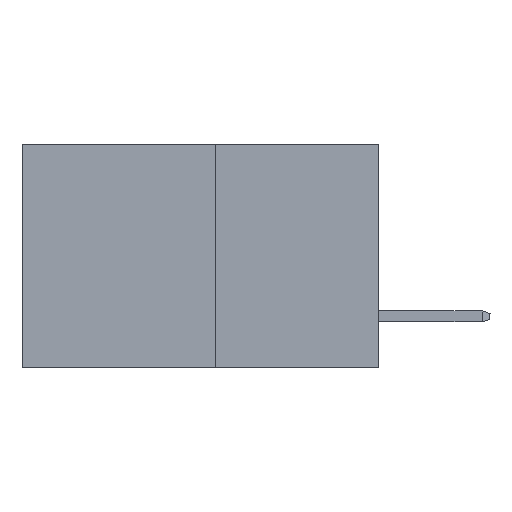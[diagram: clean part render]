
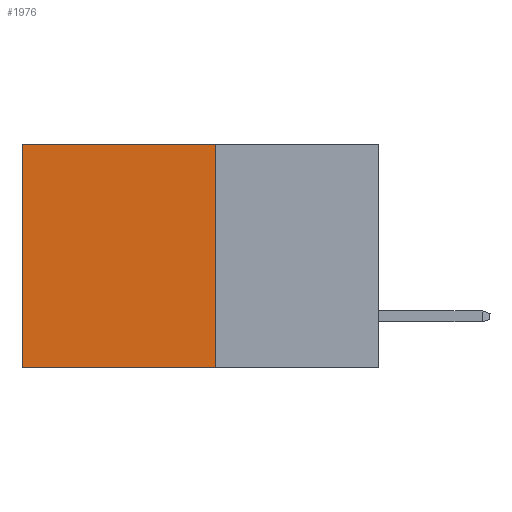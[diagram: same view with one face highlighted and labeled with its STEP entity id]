
A CAD part, left-side view. The second image highlights one B-rep face of the part: STEP entity #1976.
In plain terms, the highlighted planar face has unit normal (-1, 0, 0).
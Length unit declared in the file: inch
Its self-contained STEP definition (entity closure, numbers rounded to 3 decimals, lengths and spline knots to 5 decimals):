
#102 = AXIS2_PLACEMENT_3D ( 'NONE', #6379, #11119, #2765 ) ;
#424 = DIRECTION ( 'NONE',  ( 0., 0., -1. ) ) ;
#978 = VECTOR ( 'NONE', #2847, 39.37008 ) ;
#984 = EDGE_CURVE ( 'NONE', #10551, #9111, #11669, .T. ) ;
#1069 = VECTOR ( 'NONE', #6857, 39.37008 ) ;
#1728 = EDGE_LOOP ( 'NONE', ( #4679, #6504, #8886, #12723 ) ) ;
#1844 = VECTOR ( 'NONE', #10695, 39.37008 ) ;
#1976 = ADVANCED_FACE ( 'NONE', ( #5965 ), #11493, .F. ) ;
#2765 = DIRECTION ( 'NONE',  ( 0., 0., -1. ) ) ;
#2815 = LINE ( 'NONE', #11566, #1844 ) ;
#2847 = DIRECTION ( 'NONE',  ( 0., 1., 0. ) ) ;
#3214 = EDGE_CURVE ( 'NONE', #10551, #5088, #2815, .T. ) ;
#4679 = ORIENTED_EDGE ( 'NONE', *, *, #10017, .T. ) ;
#4968 = CARTESIAN_POINT ( 'NONE',  ( 0.277, 0.59, -0.37 ) ) ;
#5088 = VERTEX_POINT ( 'NONE', #12902 ) ;
#5836 = CARTESIAN_POINT ( 'NONE',  ( 0.277, 0.27, -0.37 ) ) ;
#5965 = FACE_OUTER_BOUND ( 'NONE', #1728, .T. ) ;
#6203 = CARTESIAN_POINT ( 'NONE',  ( 0.277, 0.59, 0. ) ) ;
#6379 = CARTESIAN_POINT ( 'NONE',  ( 0.277, 0.27, -0.37 ) ) ;
#6504 = ORIENTED_EDGE ( 'NONE', *, *, #12082, .F. ) ;
#6857 = DIRECTION ( 'NONE',  ( 0., 1., 0. ) ) ;
#8818 = LINE ( 'NONE', #5836, #1069 ) ;
#8886 = ORIENTED_EDGE ( 'NONE', *, *, #3214, .F. ) ;
#9111 = VERTEX_POINT ( 'NONE', #6203 ) ;
#9117 = VERTEX_POINT ( 'NONE', #4968 ) ;
#9477 = VECTOR ( 'NONE', #424, 39.37008 ) ;
#9798 = LINE ( 'NONE', #12445, #9477 ) ;
#10017 = EDGE_CURVE ( 'NONE', #9111, #9117, #9798, .T. ) ;
#10551 = VERTEX_POINT ( 'NONE', #12471 ) ;
#10695 = DIRECTION ( 'NONE',  ( 0., 0., -1. ) ) ;
#10715 = CARTESIAN_POINT ( 'NONE',  ( 0.277, 0.27, 0. ) ) ;
#11119 = DIRECTION ( 'NONE',  ( 1., 0., 0. ) ) ;
#11493 = PLANE ( 'NONE',  #102 ) ;
#11566 = CARTESIAN_POINT ( 'NONE',  ( 0.277, 0.27, -0.37 ) ) ;
#11669 = LINE ( 'NONE', #10715, #978 ) ;
#12082 = EDGE_CURVE ( 'NONE', #5088, #9117, #8818, .T. ) ;
#12445 = CARTESIAN_POINT ( 'NONE',  ( 0.277, 0.59, -0.37 ) ) ;
#12471 = CARTESIAN_POINT ( 'NONE',  ( 0.277, 0.27, 0. ) ) ;
#12723 = ORIENTED_EDGE ( 'NONE', *, *, #984, .T. ) ;
#12902 = CARTESIAN_POINT ( 'NONE',  ( 0.277, 0.27, -0.37 ) ) ;
